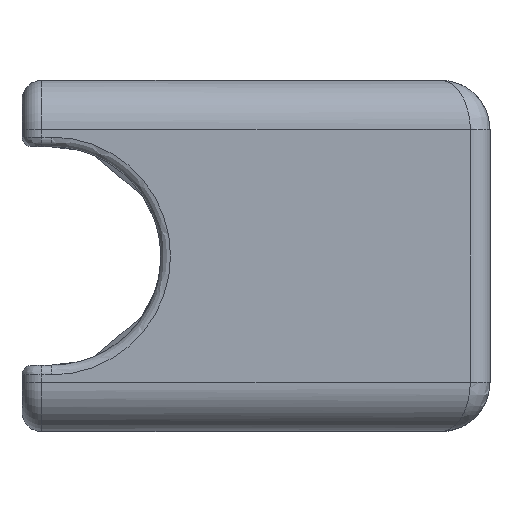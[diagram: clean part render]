
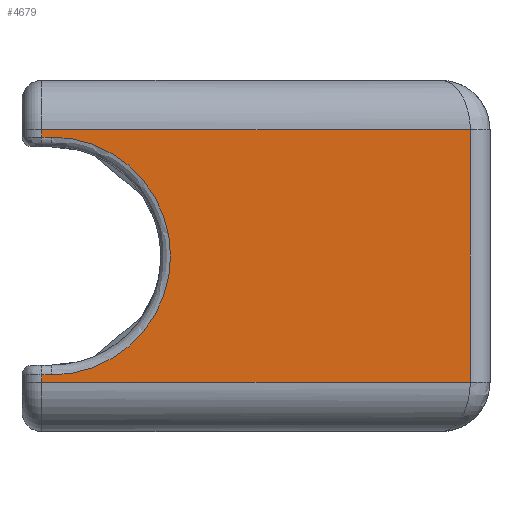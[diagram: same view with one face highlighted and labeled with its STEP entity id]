
A CAD part, left-side view. The second image highlights one B-rep face of the part: STEP entity #4679.
In plain terms, the highlighted planar face has unit normal (-1, 0, 0).
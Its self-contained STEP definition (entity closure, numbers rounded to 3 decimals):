
#89=PLANE('',#5305);
#566=FACE_OUTER_BOUND('',#876,.T.);
#876=EDGE_LOOP('',(#4048,#4049,#4050,#4051,#4052,#4053,#4054,#4055));
#1138=LINE('',#10002,#1392);
#1140=LINE('',#10070,#1394);
#1141=LINE('',#10106,#1395);
#1143=LINE('',#10113,#1397);
#1144=LINE('',#10116,#1398);
#1145=LINE('',#10118,#1399);
#1146=LINE('',#10119,#1400);
#1392=VECTOR('',#6689,10.);
#1394=VECTOR('',#6699,10.);
#1395=VECTOR('',#6714,10.);
#1397=VECTOR('',#6724,10.);
#1398=VECTOR('',#6727,10.);
#1399=VECTOR('',#6728,10.);
#1400=VECTOR('',#6729,10.);
#1751=CIRCLE('',#5291,12.016);
#2128=VERTEX_POINT('',#9991);
#2132=VERTEX_POINT('',#10000);
#2133=VERTEX_POINT('',#10054);
#2134=VERTEX_POINT('',#10068);
#2136=VERTEX_POINT('',#10099);
#2138=VERTEX_POINT('',#10109);
#2139=VERTEX_POINT('',#10115);
#2140=VERTEX_POINT('',#10117);
#2786=EDGE_CURVE('',#2132,#2128,#1138,.T.);
#2789=EDGE_CURVE('',#2133,#2132,#1751,.T.);
#2792=EDGE_CURVE('',#2134,#2133,#1140,.T.);
#2798=EDGE_CURVE('',#2128,#2136,#1141,.T.);
#2802=EDGE_CURVE('',#2138,#2134,#1143,.T.);
#2803=EDGE_CURVE('',#2139,#2138,#1144,.T.);
#2804=EDGE_CURVE('',#2140,#2139,#1145,.T.);
#2805=EDGE_CURVE('',#2136,#2140,#1146,.T.);
#4048=ORIENTED_EDGE('',*,*,#2792,.F.);
#4049=ORIENTED_EDGE('',*,*,#2802,.F.);
#4050=ORIENTED_EDGE('',*,*,#2803,.F.);
#4051=ORIENTED_EDGE('',*,*,#2804,.F.);
#4052=ORIENTED_EDGE('',*,*,#2805,.F.);
#4053=ORIENTED_EDGE('',*,*,#2798,.F.);
#4054=ORIENTED_EDGE('',*,*,#2786,.F.);
#4055=ORIENTED_EDGE('',*,*,#2789,.F.);
#4679=ADVANCED_FACE('',(#566),#89,.T.);
#5291=AXIS2_PLACEMENT_3D('',#10056,#6693,#6694);
#5305=AXIS2_PLACEMENT_3D('',#10114,#6725,#6726);
#6689=DIRECTION('',(0.,1.,0.));
#6693=DIRECTION('center_axis',(-1.,0.,0.));
#6694=DIRECTION('ref_axis',(0.,-0.868,-0.496));
#6699=DIRECTION('',(0.,-1.,0.));
#6714=DIRECTION('',(0.,0.,1.));
#6724=DIRECTION('',(0.,0.,1.));
#6725=DIRECTION('center_axis',(-1.,0.,0.));
#6726=DIRECTION('ref_axis',(0.,-1.,0.));
#6727=DIRECTION('',(0.,1.,0.));
#6728=DIRECTION('',(0.,0.,-1.));
#6729=DIRECTION('',(0.,-1.,0.));
#9991=CARTESIAN_POINT('',(-96.158,15.442,29.766));
#10000=CARTESIAN_POINT('',(-96.158,14.449,29.766));
#10002=CARTESIAN_POINT('',(-96.158,15.946,29.766));
#10054=CARTESIAN_POINT('',(-96.158,14.449,5.734));
#10056=CARTESIAN_POINT('Origin',(-96.158,14.449,17.75));
#10068=CARTESIAN_POINT('',(-96.158,15.442,5.734));
#10070=CARTESIAN_POINT('',(-96.158,17.442,5.734));
#10099=CARTESIAN_POINT('',(-96.158,15.442,30.5));
#10106=CARTESIAN_POINT('',(-96.158,15.442,0.));
#10109=CARTESIAN_POINT('',(-96.158,15.442,5.));
#10113=CARTESIAN_POINT('',(-96.158,15.442,0.));
#10114=CARTESIAN_POINT('Origin',(-96.158,17.442,0.));
#10115=CARTESIAN_POINT('',(-96.158,-27.848,5.));
#10116=CARTESIAN_POINT('',(-96.158,8.728,5.));
#10117=CARTESIAN_POINT('',(-96.158,-27.848,30.5));
#10118=CARTESIAN_POINT('',(-96.158,-27.848,17.75));
#10119=CARTESIAN_POINT('',(-96.158,8.728,30.5));
